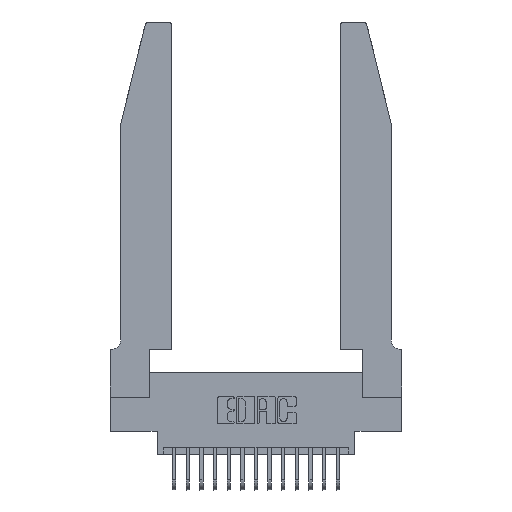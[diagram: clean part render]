
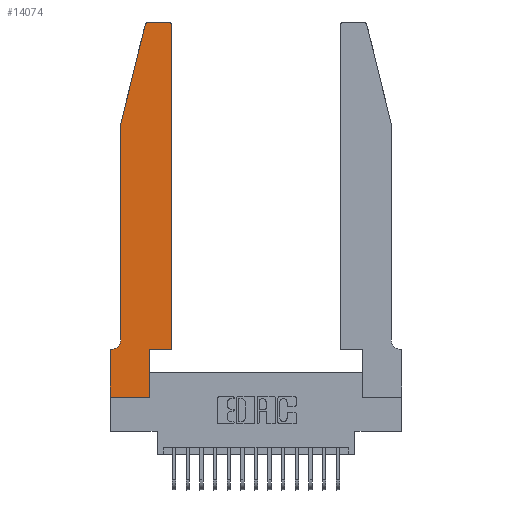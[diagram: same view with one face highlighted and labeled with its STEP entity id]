
A CAD part, top view. The second image highlights one B-rep face of the part: STEP entity #14074.
In plain terms, the highlighted planar face has unit normal (0, 0, 1).
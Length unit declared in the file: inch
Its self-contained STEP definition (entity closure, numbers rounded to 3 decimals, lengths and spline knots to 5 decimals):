
#31 = CARTESIAN_POINT ( 'NONE',  ( 0.4205, 2.75, 0.37 ) ) ;
#81 = VECTOR ( 'NONE', #20118, 39.37008 ) ;
#181 = VECTOR ( 'NONE', #8819, 39.37008 ) ;
#298 = VECTOR ( 'NONE', #12503, 39.37008 ) ;
#355 = EDGE_CURVE ( 'NONE', #19374, #7019, #14705, .T. ) ;
#385 = AXIS2_PLACEMENT_3D ( 'NONE', #8024, #18858, #9630 ) ;
#445 = ORIENTED_EDGE ( 'NONE', *, *, #355, .T. ) ;
#452 = VERTEX_POINT ( 'NONE', #6493 ) ;
#497 = EDGE_CURVE ( 'NONE', #11143, #20105, #8572, .T. ) ;
#636 = EDGE_CURVE ( 'NONE', #7019, #2836, #18978, .T. ) ;
#648 = LINE ( 'NONE', #7747, #81 ) ;
#1169 = CARTESIAN_POINT ( 'NONE',  ( 0.284, 2.75, 0.37 ) ) ;
#1290 = ORIENTED_EDGE ( 'NONE', *, *, #4983, .T. ) ;
#1446 = DIRECTION ( 'NONE',  ( 0., 0., -1. ) ) ;
#1475 = VERTEX_POINT ( 'NONE', #2245 ) ;
#2022 = AXIS2_PLACEMENT_3D ( 'NONE', #11309, #1446, #12868 ) ;
#2034 = VERTEX_POINT ( 'NONE', #12153 ) ;
#2245 = CARTESIAN_POINT ( 'NONE',  ( 0.4505, 0.35, 0.37 ) ) ;
#2273 = LINE ( 'NONE', #2900, #10522 ) ;
#2291 = DIRECTION ( 'NONE',  ( 0., 1., 0. ) ) ;
#2836 = VERTEX_POINT ( 'NONE', #9649 ) ;
#2851 = AXIS2_PLACEMENT_3D ( 'NONE', #4561, #15734, #6255 ) ;
#2900 = CARTESIAN_POINT ( 'NONE',  ( 0.2865, 0.35, 0.37 ) ) ;
#3293 = VERTEX_POINT ( 'NONE', #1169 ) ;
#3577 = CIRCLE ( 'NONE', #2022, 0.07 ) ;
#3891 = DIRECTION ( 'NONE',  ( 0., -1., 0. ) ) ;
#4458 = DIRECTION ( 'NONE',  ( 1., 0., 0. ) ) ;
#4560 = DIRECTION ( 'NONE',  ( 0., 1., 0. ) ) ;
#4561 = CARTESIAN_POINT ( 'NONE',  ( 0.284, 2.72, 0.37 ) ) ;
#4704 = ORIENTED_EDGE ( 'NONE', *, *, #20636, .T. ) ;
#4983 = EDGE_CURVE ( 'NONE', #452, #1475, #13369, .T. ) ;
#4996 = CARTESIAN_POINT ( 'NONE',  ( 0.0755, 2., 0.37 ) ) ;
#5041 = EDGE_CURVE ( 'NONE', #3293, #19374, #16025, .T. ) ;
#5270 = CARTESIAN_POINT ( 'NONE',  ( 0.4505, 2.72, 0.37 ) ) ;
#5639 = LINE ( 'NONE', #15792, #9462 ) ;
#6045 = CARTESIAN_POINT ( 'NONE',  ( 0.4505, 0.35, 0.37 ) ) ;
#6255 = DIRECTION ( 'NONE',  ( 1., 0., 0. ) ) ;
#6493 = CARTESIAN_POINT ( 'NONE',  ( 0.2865, 0.35, 0.37 ) ) ;
#6530 = VECTOR ( 'NONE', #3891, 39.37008 ) ;
#6606 = DIRECTION ( 'NONE',  ( -0.239, -0.971, 0. ) ) ;
#6789 = ORIENTED_EDGE ( 'NONE', *, *, #15504, .T. ) ;
#7019 = VERTEX_POINT ( 'NONE', #7304 ) ;
#7304 = CARTESIAN_POINT ( 'NONE',  ( 0.0755, 2., 0.37 ) ) ;
#7699 = CARTESIAN_POINT ( 'NONE',  ( 0., 0., 0.37 ) ) ;
#7747 = CARTESIAN_POINT ( 'NONE',  ( 0.0755, 0.35, 0.37 ) ) ;
#7814 = ORIENTED_EDGE ( 'NONE', *, *, #8226, .T. ) ;
#8017 = CARTESIAN_POINT ( 'NONE',  ( 0.0755, 2., 0.37 ) ) ;
#8024 = CARTESIAN_POINT ( 'NONE',  ( 0.4205, 2.72, 0.37 ) ) ;
#8226 = EDGE_CURVE ( 'NONE', #2836, #10416, #3577, .T. ) ;
#8572 = LINE ( 'NONE', #14237, #181 ) ;
#8664 = EDGE_LOOP ( 'NONE', ( #17588, #10829, #445, #12048, #7814, #15170, #11075, #6789, #10567, #1290, #17820, #4704 ) ) ;
#8819 = DIRECTION ( 'NONE',  ( 0., -1., 0. ) ) ;
#9310 = DIRECTION ( 'NONE',  ( 1., 0., 0. ) ) ;
#9366 = CARTESIAN_POINT ( 'NONE',  ( 0., 0.35, 0.37 ) ) ;
#9459 = LINE ( 'NONE', #10506, #16764 ) ;
#9462 = VECTOR ( 'NONE', #17321, 39.37008 ) ;
#9598 = EDGE_CURVE ( 'NONE', #1475, #14620, #9459, .T. ) ;
#9630 = DIRECTION ( 'NONE',  ( 1., 0., 0. ) ) ;
#9649 = CARTESIAN_POINT ( 'NONE',  ( 0.0755, 0.42, 0.37 ) ) ;
#10017 = CIRCLE ( 'NONE', #385, 0.03 ) ;
#10416 = VERTEX_POINT ( 'NONE', #11048 ) ;
#10506 = CARTESIAN_POINT ( 'NONE',  ( 0.4505, 0.35, 0.37 ) ) ;
#10522 = VECTOR ( 'NONE', #4560, 39.37008 ) ;
#10567 = ORIENTED_EDGE ( 'NONE', *, *, #13500, .T. ) ;
#10829 = ORIENTED_EDGE ( 'NONE', *, *, #5041, .T. ) ;
#11048 = CARTESIAN_POINT ( 'NONE',  ( 0.0055, 0.35, 0.37 ) ) ;
#11075 = ORIENTED_EDGE ( 'NONE', *, *, #497, .T. ) ;
#11143 = VERTEX_POINT ( 'NONE', #11160 ) ;
#11160 = CARTESIAN_POINT ( 'NONE',  ( 0., 0.35, 0.37 ) ) ;
#11309 = CARTESIAN_POINT ( 'NONE',  ( 0.0055, 0.42, 0.37 ) ) ;
#11343 = VERTEX_POINT ( 'NONE', #31 ) ;
#11752 = CARTESIAN_POINT ( 'NONE',  ( 0.25487, 2.72718, 0.37 ) ) ;
#12048 = ORIENTED_EDGE ( 'NONE', *, *, #636, .T. ) ;
#12153 = CARTESIAN_POINT ( 'NONE',  ( 0.2865, 0., 0.37 ) ) ;
#12503 = DIRECTION ( 'NONE',  ( 1., 0., 0. ) ) ;
#12544 = PLANE ( 'NONE',  #18750 ) ;
#12767 = CARTESIAN_POINT ( 'NONE',  ( 0., 0., 0.37 ) ) ;
#12868 = DIRECTION ( 'NONE',  ( -1., 0., 0. ) ) ;
#13369 = LINE ( 'NONE', #6045, #298 ) ;
#13500 = EDGE_CURVE ( 'NONE', #2034, #452, #2273, .T. ) ;
#14057 = EDGE_CURVE ( 'NONE', #10416, #11143, #648, .T. ) ;
#14074 = ADVANCED_FACE ( 'NONE', ( #16802 ), #12544, .T. ) ;
#14090 = DIRECTION ( 'NONE',  ( 0., 0., 1. ) ) ;
#14237 = CARTESIAN_POINT ( 'NONE',  ( 0., 0., 0.37 ) ) ;
#14620 = VERTEX_POINT ( 'NONE', #5270 ) ;
#14705 = LINE ( 'NONE', #4996, #19208 ) ;
#15170 = ORIENTED_EDGE ( 'NONE', *, *, #14057, .T. ) ;
#15504 = EDGE_CURVE ( 'NONE', #20105, #2034, #16056, .T. ) ;
#15596 = EDGE_CURVE ( 'NONE', #11343, #3293, #5639, .T. ) ;
#15734 = DIRECTION ( 'NONE',  ( 0., 0., 1. ) ) ;
#15792 = CARTESIAN_POINT ( 'NONE',  ( 0.2605, 2.75, 0.37 ) ) ;
#16025 = CIRCLE ( 'NONE', #2851, 0.03 ) ;
#16056 = LINE ( 'NONE', #7699, #19577 ) ;
#16764 = VECTOR ( 'NONE', #2291, 39.37008 ) ;
#16802 = FACE_OUTER_BOUND ( 'NONE', #8664, .T. ) ;
#17321 = DIRECTION ( 'NONE',  ( -1., 0., 0. ) ) ;
#17588 = ORIENTED_EDGE ( 'NONE', *, *, #15596, .T. ) ;
#17820 = ORIENTED_EDGE ( 'NONE', *, *, #9598, .T. ) ;
#18750 = AXIS2_PLACEMENT_3D ( 'NONE', #9366, #14090, #4458 ) ;
#18858 = DIRECTION ( 'NONE',  ( 0., 0., 1. ) ) ;
#18978 = LINE ( 'NONE', #8017, #6530 ) ;
#19208 = VECTOR ( 'NONE', #6606, 39.37008 ) ;
#19374 = VERTEX_POINT ( 'NONE', #11752 ) ;
#19577 = VECTOR ( 'NONE', #9310, 39.37008 ) ;
#20105 = VERTEX_POINT ( 'NONE', #12767 ) ;
#20118 = DIRECTION ( 'NONE',  ( -1., 0., 0. ) ) ;
#20636 = EDGE_CURVE ( 'NONE', #14620, #11343, #10017, .T. ) ;
